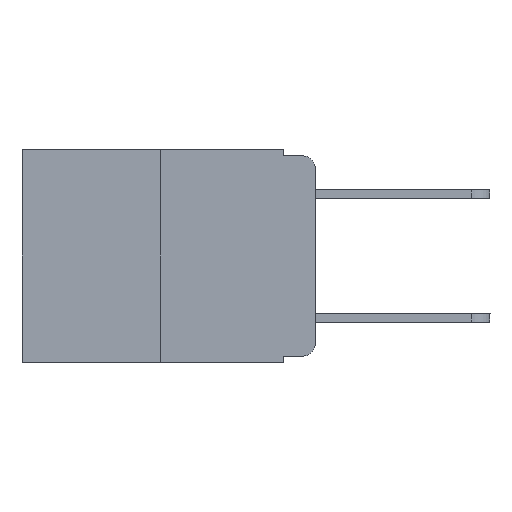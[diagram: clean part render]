
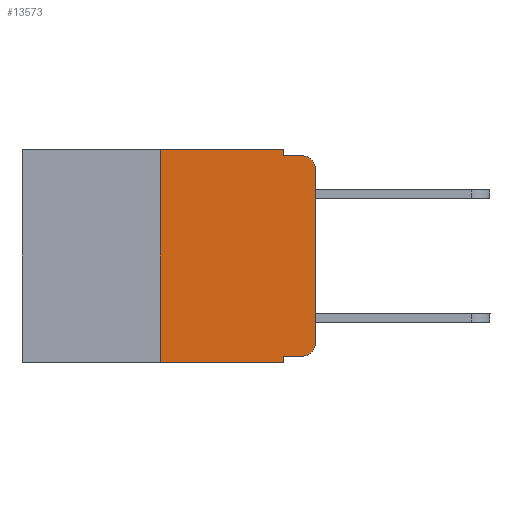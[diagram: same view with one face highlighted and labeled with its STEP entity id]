
A CAD part, left-side view. The second image highlights one B-rep face of the part: STEP entity #13573.
In plain terms, the highlighted planar face has unit normal (-1, 0, 0).
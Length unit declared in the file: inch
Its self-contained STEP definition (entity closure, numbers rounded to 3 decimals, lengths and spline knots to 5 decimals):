
#4 = CARTESIAN_POINT ( 'NONE',  ( 0., 0.25, 0. ) ) ;
#146 = VERTEX_POINT ( 'NONE', #4 ) ;
#609 = AXIS2_PLACEMENT_3D ( 'NONE', #11854, #3452, #13024 ) ;
#697 = ORIENTED_EDGE ( 'NONE', *, *, #10957, .F. ) ;
#857 = VECTOR ( 'NONE', #15430, 39.37008 ) ;
#1340 = CARTESIAN_POINT ( 'NONE',  ( 0., 0.051, -0.333 ) ) ;
#1356 = CARTESIAN_POINT ( 'NONE',  ( 0., 0.051, -0.01 ) ) ;
#1408 = EDGE_CURVE ( 'NONE', #8275, #146, #13926, .T. ) ;
#1505 = CARTESIAN_POINT ( 'NONE',  ( 0., 0.051, 0. ) ) ;
#1828 = VERTEX_POINT ( 'NONE', #12406 ) ;
#1874 = ORIENTED_EDGE ( 'NONE', *, *, #4911, .T. ) ;
#1946 = CARTESIAN_POINT ( 'NONE',  ( 0., 0.02, -0.313 ) ) ;
#1965 = EDGE_CURVE ( 'NONE', #12524, #10044, #6970, .T. ) ;
#1994 = DIRECTION ( 'NONE',  ( 0., -1., 0. ) ) ;
#2104 = CARTESIAN_POINT ( 'NONE',  ( 0., 0.473, -0.343 ) ) ;
#2187 = ORIENTED_EDGE ( 'NONE', *, *, #1408, .F. ) ;
#2326 = CARTESIAN_POINT ( 'NONE',  ( 0., 0.25, -0.343 ) ) ;
#2608 = LINE ( 'NONE', #1356, #10153 ) ;
#2830 = EDGE_CURVE ( 'NONE', #9701, #9693, #15192, .T. ) ;
#3184 = DIRECTION ( 'NONE',  ( 0., 0., -1. ) ) ;
#3275 = CARTESIAN_POINT ( 'NONE',  ( 0., 0., -0.313 ) ) ;
#3412 = CARTESIAN_POINT ( 'NONE',  ( 0., 0.473, 0. ) ) ;
#3452 = DIRECTION ( 'NONE',  ( -1., 0., 0. ) ) ;
#3512 = CARTESIAN_POINT ( 'NONE',  ( 0., 0., -0.03 ) ) ;
#3619 = VECTOR ( 'NONE', #3757, 39.37008 ) ;
#3757 = DIRECTION ( 'NONE',  ( 0., 0., -1. ) ) ;
#4141 = CARTESIAN_POINT ( 'NONE',  ( 0., 0.051, -0.343 ) ) ;
#4247 = DIRECTION ( 'NONE',  ( 0., 0., 1. ) ) ;
#4684 = CARTESIAN_POINT ( 'NONE',  ( 0., 0.051, 0. ) ) ;
#4911 = EDGE_CURVE ( 'NONE', #1828, #11701, #8585, .T. ) ;
#5441 = VECTOR ( 'NONE', #13104, 39.37008 ) ;
#5473 = VECTOR ( 'NONE', #4247, 39.37008 ) ;
#5662 = VECTOR ( 'NONE', #1994, 39.37008 ) ;
#6214 = DIRECTION ( 'NONE',  ( 0., -1., 0. ) ) ;
#6249 = VERTEX_POINT ( 'NONE', #4141 ) ;
#6762 = EDGE_CURVE ( 'NONE', #10336, #9701, #9066, .T. ) ;
#6970 = LINE ( 'NONE', #4684, #5441 ) ;
#7165 = AXIS2_PLACEMENT_3D ( 'NONE', #1946, #8099, #3184 ) ;
#7467 = CARTESIAN_POINT ( 'NONE',  ( 0., 0.051, -0.01 ) ) ;
#7469 = ORIENTED_EDGE ( 'NONE', *, *, #13923, .F. ) ;
#8012 = ORIENTED_EDGE ( 'NONE', *, *, #1965, .F. ) ;
#8029 = CARTESIAN_POINT ( 'NONE',  ( 0., 0.473, 0. ) ) ;
#8099 = DIRECTION ( 'NONE',  ( -1., 0., 0. ) ) ;
#8275 = VERTEX_POINT ( 'NONE', #2326 ) ;
#8585 = LINE ( 'NONE', #1340, #14568 ) ;
#8889 = LINE ( 'NONE', #2104, #5662 ) ;
#8917 = CARTESIAN_POINT ( 'NONE',  ( 0., 0.051, 0. ) ) ;
#8928 = CARTESIAN_POINT ( 'NONE',  ( 0., 0., 0. ) ) ;
#9066 = LINE ( 'NONE', #8928, #13210 ) ;
#9085 = DIRECTION ( 'NONE',  ( 1., 0., 0. ) ) ;
#9151 = ORIENTED_EDGE ( 'NONE', *, *, #14854, .T. ) ;
#9204 = EDGE_CURVE ( 'NONE', #10044, #9693, #2608, .T. ) ;
#9528 = EDGE_CURVE ( 'NONE', #11701, #10336, #10498, .T. ) ;
#9693 = VERTEX_POINT ( 'NONE', #10543 ) ;
#9701 = VERTEX_POINT ( 'NONE', #3512 ) ;
#10044 = VERTEX_POINT ( 'NONE', #7467 ) ;
#10153 = VECTOR ( 'NONE', #6214, 39.37008 ) ;
#10336 = VERTEX_POINT ( 'NONE', #3275 ) ;
#10437 = ORIENTED_EDGE ( 'NONE', *, *, #6762, .T. ) ;
#10498 = CIRCLE ( 'NONE', #7165, 0.02 ) ;
#10543 = CARTESIAN_POINT ( 'NONE',  ( 0., 0.02, -0.01 ) ) ;
#10849 = CARTESIAN_POINT ( 'NONE',  ( 0., 0.02, -0.333 ) ) ;
#10957 = EDGE_CURVE ( 'NONE', #146, #12524, #14604, .T. ) ;
#11207 = ORIENTED_EDGE ( 'NONE', *, *, #9528, .T. ) ;
#11304 = DIRECTION ( 'NONE',  ( 0., 0., 1. ) ) ;
#11520 = PLANE ( 'NONE',  #14467 ) ;
#11701 = VERTEX_POINT ( 'NONE', #10849 ) ;
#11854 = CARTESIAN_POINT ( 'NONE',  ( 0., 0.02, -0.03 ) ) ;
#12406 = CARTESIAN_POINT ( 'NONE',  ( 0., 0.051, -0.333 ) ) ;
#12468 = FACE_OUTER_BOUND ( 'NONE', #12545, .T. ) ;
#12524 = VERTEX_POINT ( 'NONE', #8917 ) ;
#12545 = EDGE_LOOP ( 'NONE', ( #10437, #15068, #13868, #8012, #697, #2187, #9151, #7469, #1874, #11207 ) ) ;
#13024 = DIRECTION ( 'NONE',  ( 0., 0., -1. ) ) ;
#13104 = DIRECTION ( 'NONE',  ( 0., 0., -1. ) ) ;
#13210 = VECTOR ( 'NONE', #11304, 39.37008 ) ;
#13410 = DIRECTION ( 'NONE',  ( 0., -1., 0. ) ) ;
#13573 = ADVANCED_FACE ( 'NONE', ( #12468 ), #11520, .F. ) ;
#13868 = ORIENTED_EDGE ( 'NONE', *, *, #9204, .F. ) ;
#13923 = EDGE_CURVE ( 'NONE', #1828, #6249, #14506, .T. ) ;
#13926 = LINE ( 'NONE', #14521, #5473 ) ;
#13990 = DIRECTION ( 'NONE',  ( 0., 0., -1. ) ) ;
#14467 = AXIS2_PLACEMENT_3D ( 'NONE', #8029, #9085, #13990 ) ;
#14506 = LINE ( 'NONE', #1505, #3619 ) ;
#14521 = CARTESIAN_POINT ( 'NONE',  ( 0., 0.25, 0. ) ) ;
#14568 = VECTOR ( 'NONE', #13410, 39.37008 ) ;
#14604 = LINE ( 'NONE', #3412, #857 ) ;
#14854 = EDGE_CURVE ( 'NONE', #8275, #6249, #8889, .T. ) ;
#15068 = ORIENTED_EDGE ( 'NONE', *, *, #2830, .T. ) ;
#15192 = CIRCLE ( 'NONE', #609, 0.02 ) ;
#15430 = DIRECTION ( 'NONE',  ( 0., -1., 0. ) ) ;
